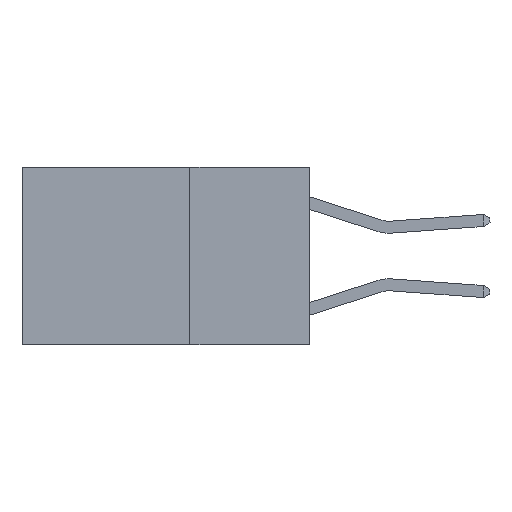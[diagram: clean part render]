
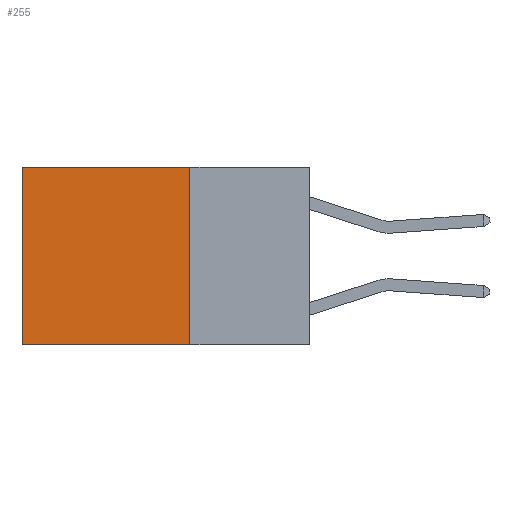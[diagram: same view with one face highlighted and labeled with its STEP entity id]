
A CAD part, left-side view. The second image highlights one B-rep face of the part: STEP entity #255.
In plain terms, the highlighted planar face has unit normal (-1, 0, 0).
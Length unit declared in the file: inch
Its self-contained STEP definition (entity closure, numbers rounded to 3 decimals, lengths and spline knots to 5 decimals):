
#255 = ADVANCED_FACE ( 'NONE', ( #3660 ), #12455, .F. ) ;
#526 = AXIS2_PLACEMENT_3D ( 'NONE', #12292, #11030, #11185 ) ;
#1462 = CARTESIAN_POINT ( 'NONE',  ( 0.2625, 0.6, 0. ) ) ;
#2039 = CARTESIAN_POINT ( 'NONE',  ( 0.2625, 0.25, 0. ) ) ;
#2134 = ORIENTED_EDGE ( 'NONE', *, *, #6008, .T. ) ;
#2388 = LINE ( 'NONE', #12644, #11229 ) ;
#2867 = VERTEX_POINT ( 'NONE', #9173 ) ;
#3094 = EDGE_CURVE ( 'NONE', #10290, #2867, #10136, .T. ) ;
#3660 = FACE_OUTER_BOUND ( 'NONE', #11906, .T. ) ;
#3847 = ORIENTED_EDGE ( 'NONE', *, *, #3094, .F. ) ;
#4581 = VERTEX_POINT ( 'NONE', #10963 ) ;
#4697 = EDGE_CURVE ( 'NONE', #9520, #2867, #9914, .T. ) ;
#5804 = CARTESIAN_POINT ( 'NONE',  ( 0.2625, 0.25, -0.37 ) ) ;
#6008 = EDGE_CURVE ( 'NONE', #4581, #9520, #2388, .T. ) ;
#6210 = VECTOR ( 'NONE', #7009, 39.37008 ) ;
#6250 = LINE ( 'NONE', #2039, #11681 ) ;
#6840 = DIRECTION ( 'NONE',  ( 0., 0., -1. ) ) ;
#6994 = CARTESIAN_POINT ( 'NONE',  ( 0.2625, 0.25, -0.37 ) ) ;
#7009 = DIRECTION ( 'NONE',  ( 0., 1., 0. ) ) ;
#9173 = CARTESIAN_POINT ( 'NONE',  ( 0.2625, 0.6, -0.37 ) ) ;
#9193 = ORIENTED_EDGE ( 'NONE', *, *, #9879, .F. ) ;
#9520 = VERTEX_POINT ( 'NONE', #1462 ) ;
#9879 = EDGE_CURVE ( 'NONE', #4581, #10290, #6250, .T. ) ;
#9914 = LINE ( 'NONE', #12647, #15579 ) ;
#10136 = LINE ( 'NONE', #5804, #6210 ) ;
#10290 = VERTEX_POINT ( 'NONE', #6994 ) ;
#10681 = DIRECTION ( 'NONE',  ( 0., 1., 0. ) ) ;
#10963 = CARTESIAN_POINT ( 'NONE',  ( 0.2625, 0.25, 0. ) ) ;
#11030 = DIRECTION ( 'NONE',  ( 1., 0., 0. ) ) ;
#11185 = DIRECTION ( 'NONE',  ( 0., 0., -1. ) ) ;
#11229 = VECTOR ( 'NONE', #10681, 39.37008 ) ;
#11265 = DIRECTION ( 'NONE',  ( 0., 0., -1. ) ) ;
#11681 = VECTOR ( 'NONE', #6840, 39.37008 ) ;
#11906 = EDGE_LOOP ( 'NONE', ( #14822, #3847, #9193, #2134 ) ) ;
#12292 = CARTESIAN_POINT ( 'NONE',  ( 0.2625, 0.25, 0. ) ) ;
#12455 = PLANE ( 'NONE',  #526 ) ;
#12644 = CARTESIAN_POINT ( 'NONE',  ( 0.2625, 0.25, 0. ) ) ;
#12647 = CARTESIAN_POINT ( 'NONE',  ( 0.2625, 0.6, 0. ) ) ;
#14822 = ORIENTED_EDGE ( 'NONE', *, *, #4697, .T. ) ;
#15579 = VECTOR ( 'NONE', #11265, 39.37008 ) ;
